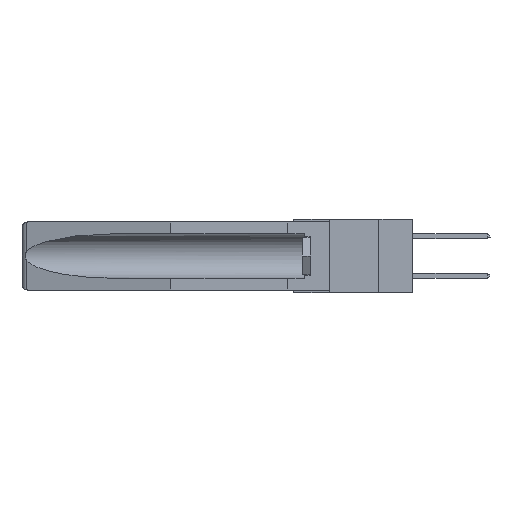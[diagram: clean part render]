
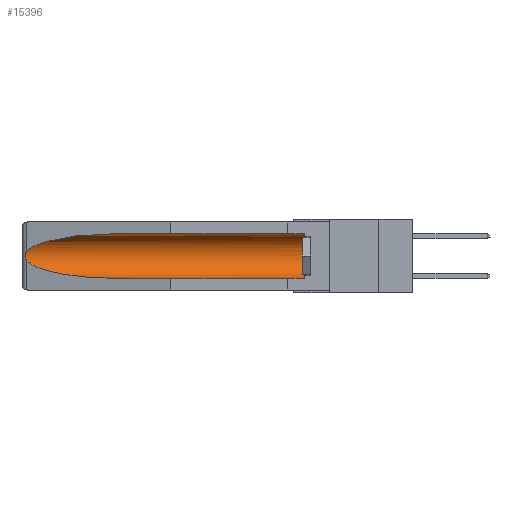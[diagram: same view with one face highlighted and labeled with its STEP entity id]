
A CAD part, left-side view. The second image highlights one B-rep face of the part: STEP entity #15396.
In plain terms, the highlighted cylindrical face has radius 2.857 mm (diameter 5.715 mm), a partial arc.
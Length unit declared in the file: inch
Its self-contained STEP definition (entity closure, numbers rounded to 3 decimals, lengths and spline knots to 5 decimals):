
#197 = CARTESIAN_POINT ( 'NONE',  ( 0.155, 1.07973, -0.284 ) ) ;
#782 = CARTESIAN_POINT ( 'NONE',  ( 0.2673, 1.53269, -0.17917 ) ) ;
#1422 = CARTESIAN_POINT ( 'NONE',  ( 0.155, 1.07973, -0.059 ) ) ;
#1939 = CARTESIAN_POINT ( 'NONE',  ( 0.26597, 1.52961, -0.15275 ) ) ;
#2199 = CARTESIAN_POINT ( 'NONE',  ( 0.21114, 1.30732, -0.059 ) ) ;
#2205 = CARTESIAN_POINT ( 'NONE',  ( 0.26655, 1.53094, -0.18657 ) ) ;
#2476 = VECTOR ( 'NONE', #5025, 39.37008 ) ;
#3180 = ORIENTED_EDGE ( 'NONE', *, *, #9573, .T. ) ;
#3239 = ORIENTED_EDGE ( 'NONE', *, *, #12453, .T. ) ;
#3294 = CARTESIAN_POINT ( 'NONE',  ( 0.155, -0.30754, -0.059 ) ) ;
#3312 = CARTESIAN_POINT ( 'NONE',  ( 0.26537, 1.52718, -0.14972 ) ) ;
#3451 = ORIENTED_EDGE ( 'NONE', *, *, #10504, .T. ) ;
#3701 = CARTESIAN_POINT ( 'NONE',  ( 0.2675, 1.53308, -0.17534 ) ) ;
#4015 = B_SPLINE_CURVE_WITH_KNOTS ( 'NONE', 3,
 ( #3312, #1939, #18364, #16915, #5243, #3701, #782, #2205, #18978, #6907 ),
 .UNSPECIFIED., .F., .F.,
 ( 4, 2, 2, 2, 4 ),
 ( 0., 0.00029, 0.00058, 0.00087, 0.00117 ),
 .UNSPECIFIED. ) ;
#4730 = CARTESIAN_POINT ( 'NONE',  ( 0.26537, 1.52718, -0.19328 ) ) ;
#5007 = DIRECTION ( 'NONE',  ( 0., 1., 0. ) ) ;
#5025 = DIRECTION ( 'NONE',  ( 0., 1., 0. ) ) ;
#5170 = ORIENTED_EDGE ( 'NONE', *, *, #6168, .T. ) ;
#5243 = CARTESIAN_POINT ( 'NONE',  ( 0.2675, 1.53308, -0.16763 ) ) ;
#5488 =( BOUNDED_CURVE ( )  B_SPLINE_CURVE ( 3, ( #4730, #10777, #15301, #197 ),
 .UNSPECIFIED., .F., .F. ) 
 B_SPLINE_CURVE_WITH_KNOTS ( ( 4, 4 ),
 ( 0.1948, 1.5708 ),
 .UNSPECIFIED. ) 
 CURVE ( )  GEOMETRIC_REPRESENTATION_ITEM ( )  RATIONAL_B_SPLINE_CURVE ( ( 1., 0.848, 0.848, 1. ) ) 
 REPRESENTATION_ITEM ( '' )  );
#5660 = AXIS2_PLACEMENT_3D ( 'NONE', #12767, #15790, #18861 ) ;
#6105 = ORIENTED_EDGE ( 'NONE', *, *, #6770, .F. ) ;
#6168 = EDGE_CURVE ( 'NONE', #7706, #12415, #5488, .T. ) ;
#6618 = VERTEX_POINT ( 'NONE', #9365 ) ;
#6770 = EDGE_CURVE ( 'NONE', #7346, #12415, #9698, .T. ) ;
#6860 = CYLINDRICAL_SURFACE ( 'NONE', #8732, 0.1125 ) ;
#6907 = CARTESIAN_POINT ( 'NONE',  ( 0.26537, 1.52718, -0.19328 ) ) ;
#7002 = CARTESIAN_POINT ( 'NONE',  ( 0.26537, 1.52718, -0.19328 ) ) ;
#7346 = VERTEX_POINT ( 'NONE', #17369 ) ;
#7706 = VERTEX_POINT ( 'NONE', #7002 ) ;
#7869 = CARTESIAN_POINT ( 'NONE',  ( 0.155, -0.30754, -0.284 ) ) ;
#8233 = CARTESIAN_POINT ( 'NONE',  ( 0.26537, 1.52718, -0.14972 ) ) ;
#8732 = AXIS2_PLACEMENT_3D ( 'NONE', #17823, #10348, #14920 ) ;
#9365 = CARTESIAN_POINT ( 'NONE',  ( 0.26537, 1.52718, -0.14972 ) ) ;
#9573 = EDGE_CURVE ( 'NONE', #6618, #7706, #4015, .T. ) ;
#9608 = LINE ( 'NONE', #3294, #2476 ) ;
#9678 = VERTEX_POINT ( 'NONE', #9764 ) ;
#9698 = LINE ( 'NONE', #7869, #17273 ) ;
#9764 = CARTESIAN_POINT ( 'NONE',  ( 0.155, 1.07973, -0.059 ) ) ;
#10003 = CIRCLE ( 'NONE', #5660, 0.1125 ) ;
#10025 = EDGE_CURVE ( 'NONE', #9678, #6618, #11296, .T. ) ;
#10348 = DIRECTION ( 'NONE',  ( 0., 1., 0. ) ) ;
#10504 = EDGE_CURVE ( 'NONE', #16789, #9678, #9608, .T. ) ;
#10777 = CARTESIAN_POINT ( 'NONE',  ( 0.25451, 1.48313, -0.24835 ) ) ;
#11269 = CARTESIAN_POINT ( 'NONE',  ( 0.155, 1.07973, -0.284 ) ) ;
#11296 =( BOUNDED_CURVE ( )  B_SPLINE_CURVE ( 3, ( #1422, #2199, #15903, #8233 ),
 .UNSPECIFIED., .F., .F. ) 
 B_SPLINE_CURVE_WITH_KNOTS ( ( 4, 4 ),
 ( 4.71239, 6.08839 ),
 .UNSPECIFIED. ) 
 CURVE ( )  GEOMETRIC_REPRESENTATION_ITEM ( )  RATIONAL_B_SPLINE_CURVE ( ( 1., 0.848, 0.848, 1. ) ) 
 REPRESENTATION_ITEM ( '' )  );
#11697 = EDGE_LOOP ( 'NONE', ( #15449, #3180, #5170, #6105, #3239, #3451 ) ) ;
#12415 = VERTEX_POINT ( 'NONE', #11269 ) ;
#12453 = EDGE_CURVE ( 'NONE', #7346, #16789, #10003, .T. ) ;
#12767 = CARTESIAN_POINT ( 'NONE',  ( 0.155, 0.126, -0.1715 ) ) ;
#14920 = DIRECTION ( 'NONE',  ( 0., 0., 1. ) ) ;
#15301 = CARTESIAN_POINT ( 'NONE',  ( 0.21114, 1.30732, -0.284 ) ) ;
#15352 = FACE_OUTER_BOUND ( 'NONE', #11697, .T. ) ;
#15396 = ADVANCED_FACE ( 'NONE', ( #15352 ), #6860, .F. ) ;
#15449 = ORIENTED_EDGE ( 'NONE', *, *, #10025, .T. ) ;
#15790 = DIRECTION ( 'NONE',  ( 0., -1., 0. ) ) ;
#15903 = CARTESIAN_POINT ( 'NONE',  ( 0.25451, 1.48313, -0.09465 ) ) ;
#16789 = VERTEX_POINT ( 'NONE', #18053 ) ;
#16915 = CARTESIAN_POINT ( 'NONE',  ( 0.2673, 1.5327, -0.16383 ) ) ;
#17273 = VECTOR ( 'NONE', #5007, 39.37008 ) ;
#17369 = CARTESIAN_POINT ( 'NONE',  ( 0.155, 0.126, -0.284 ) ) ;
#17823 = CARTESIAN_POINT ( 'NONE',  ( 0.155, -0.30754, -0.1715 ) ) ;
#18053 = CARTESIAN_POINT ( 'NONE',  ( 0.155, 0.126, -0.059 ) ) ;
#18364 = CARTESIAN_POINT ( 'NONE',  ( 0.26654, 1.53092, -0.15636 ) ) ;
#18861 = DIRECTION ( 'NONE',  ( 0., 0., 1. ) ) ;
#18978 = CARTESIAN_POINT ( 'NONE',  ( 0.26597, 1.5296, -0.19026 ) ) ;
